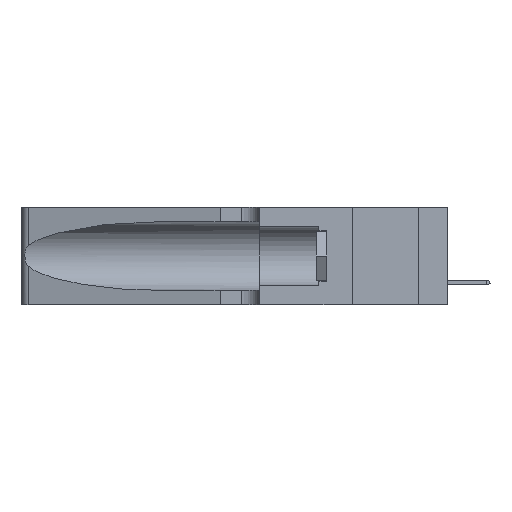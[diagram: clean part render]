
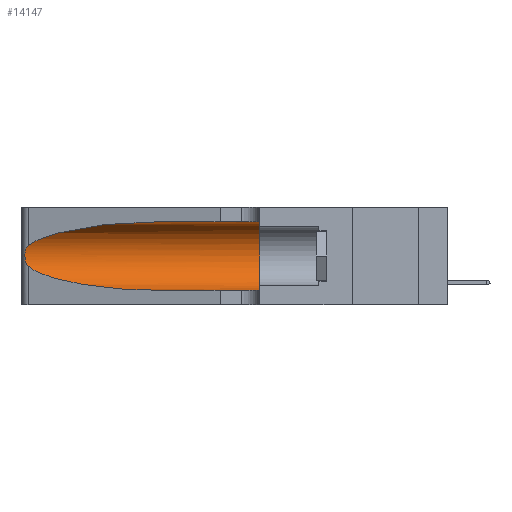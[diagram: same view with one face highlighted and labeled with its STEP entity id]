
A CAD part, left-side view. The second image highlights one B-rep face of the part: STEP entity #14147.
In plain terms, the highlighted cylindrical face has radius 3.308 mm (diameter 6.617 mm), a partial arc.
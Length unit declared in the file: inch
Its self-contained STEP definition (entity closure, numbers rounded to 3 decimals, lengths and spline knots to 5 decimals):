
#588 = VERTEX_POINT ( 'NONE', #4033 ) ;
#1008 = AXIS2_PLACEMENT_3D ( 'NONE', #1620, #20539, #9808 ) ;
#1588 = CARTESIAN_POINT ( 'NONE',  ( 0.18966, 0.96281, 0.05475 ) ) ;
#1620 = CARTESIAN_POINT ( 'NONE',  ( 0.1305, 1.61858, 0.185 ) ) ;
#1772 = ORIENTED_EDGE ( 'NONE', *, *, #20546, .T. ) ;
#1859 = EDGE_LOOP ( 'NONE', ( #26863, #9785, #7416, #1772, #9924, #25585 ) ) ;
#1901 = EDGE_CURVE ( 'NONE', #8899, #8452, #25184, .T. ) ;
#2953 = CARTESIAN_POINT ( 'NONE',  ( 0.25487, 1.22718, 0.22369 ) ) ;
#4033 = CARTESIAN_POINT ( 'NONE',  ( 0.1305, 0.35, 0.05475 ) ) ;
#4034 = VERTEX_POINT ( 'NONE', #15473 ) ;
#4769 = DIRECTION ( 'NONE',  ( 0., -1., 0. ) ) ;
#5078 = CARTESIAN_POINT ( 'NONE',  ( 0.25555, 1.22994, 0.2215 ) ) ;
#5127 = VECTOR ( 'NONE', #4769, 39.37008 ) ;
#5236 = DIRECTION ( 'NONE',  ( 0., 0., 1. ) ) ;
#5252 = CARTESIAN_POINT ( 'NONE',  ( 0.26075, 1.23896, 0.19203 ) ) ;
#5438 =( BOUNDED_CURVE ( )  B_SPLINE_CURVE ( 3, ( #11975, #26789, #1588, #12551 ),
 .UNSPECIFIED., .F., .T. ) 
 B_SPLINE_CURVE_WITH_KNOTS ( ( 4, 4 ),
 ( 3.44316, 4.71239 ),
 .UNSPECIFIED. ) 
 CURVE ( )  GEOMETRIC_REPRESENTATION_ITEM ( )  RATIONAL_B_SPLINE_CURVE ( ( 1., 0.87, 0.87, 1. ) ) 
 REPRESENTATION_ITEM ( '' )  );
#5460 = CARTESIAN_POINT ( 'NONE',  ( 0.25487, 1.22718, 0.22369 ) ) ;
#5530 = CARTESIAN_POINT ( 'NONE',  ( 0.25789, 1.23486, 0.15765 ) ) ;
#6013 = CARTESIAN_POINT ( 'NONE',  ( 0.25487, 1.22718, 0.22369 ) ) ;
#6825 = CARTESIAN_POINT ( 'NONE',  ( 0.1305, 0.72297, 0.05475 ) ) ;
#7416 = ORIENTED_EDGE ( 'NONE', *, *, #7505, .T. ) ;
#7505 = EDGE_CURVE ( 'NONE', #4034, #18145, #5438, .T. ) ;
#7836 =( BOUNDED_CURVE ( )  B_SPLINE_CURVE ( 3, ( #18072, #12247, #9733, #5460 ),
 .UNSPECIFIED., .F., .F. ) 
 B_SPLINE_CURVE_WITH_KNOTS ( ( 4, 4 ),
 ( 1.5708, 2.84003 ),
 .UNSPECIFIED. ) 
 CURVE ( )  GEOMETRIC_REPRESENTATION_ITEM ( )  RATIONAL_B_SPLINE_CURVE ( ( 1., 0.87, 0.87, 1. ) ) 
 REPRESENTATION_ITEM ( '' )  );
#8098 = CARTESIAN_POINT ( 'NONE',  ( 0.1305, 1.61858, 0.31525 ) ) ;
#8452 = VERTEX_POINT ( 'NONE', #18355 ) ;
#8899 = VERTEX_POINT ( 'NONE', #20578 ) ;
#9327 = CARTESIAN_POINT ( 'NONE',  ( 0.26018, 1.23835, 0.19895 ) ) ;
#9733 = CARTESIAN_POINT ( 'NONE',  ( 0.2373, 1.15595, 0.28018 ) ) ;
#9785 = ORIENTED_EDGE ( 'NONE', *, *, #19015, .T. ) ;
#9808 = DIRECTION ( 'NONE',  ( 0., 0., -1. ) ) ;
#9924 = ORIENTED_EDGE ( 'NONE', *, *, #17853, .F. ) ;
#11975 = CARTESIAN_POINT ( 'NONE',  ( 0.25487, 1.22718, 0.14631 ) ) ;
#12247 = CARTESIAN_POINT ( 'NONE',  ( 0.18966, 0.96281, 0.31525 ) ) ;
#12551 = CARTESIAN_POINT ( 'NONE',  ( 0.1305, 0.72297, 0.05475 ) ) ;
#13292 = CARTESIAN_POINT ( 'NONE',  ( 0.1305, 1.61858, 0.05475 ) ) ;
#13763 = CARTESIAN_POINT ( 'NONE',  ( 0.26017, 1.23833, 0.17102 ) ) ;
#14098 = DIRECTION ( 'NONE',  ( 0., -1., 0. ) ) ;
#14147 = ADVANCED_FACE ( 'NONE', ( #22108 ), #26999, .F. ) ;
#15473 = CARTESIAN_POINT ( 'NONE',  ( 0.25487, 1.22718, 0.14631 ) ) ;
#15841 = CARTESIAN_POINT ( 'NONE',  ( 0.25856, 1.23593, 0.16098 ) ) ;
#17234 = B_SPLINE_CURVE_WITH_KNOTS ( 'NONE', 3,
 ( #2953, #5078, #19810, #24023, #21923, #9327, #5252, #26278, #13763, #15841, #5530, #22568, #18411, #22476 ),
 .UNSPECIFIED., .F., .F.,
 ( 4, 2, 2, 2, 2, 2, 4 ),
 ( 0., 0.00027, 0.00053, 0.00107, 0.0016, 0.00187, 0.00214 ),
 .UNSPECIFIED. ) ;
#17290 = CIRCLE ( 'NONE', #20095, 0.13025 ) ;
#17853 = EDGE_CURVE ( 'NONE', #8452, #588, #17290, .T. ) ;
#18072 = CARTESIAN_POINT ( 'NONE',  ( 0.1305, 0.72297, 0.31525 ) ) ;
#18145 = VERTEX_POINT ( 'NONE', #6825 ) ;
#18355 = CARTESIAN_POINT ( 'NONE',  ( 0.1305, 0.35, 0.31525 ) ) ;
#18411 = CARTESIAN_POINT ( 'NONE',  ( 0.25555, 1.22993, 0.14849 ) ) ;
#19015 = EDGE_CURVE ( 'NONE', #24455, #4034, #17234, .T. ) ;
#19283 = LINE ( 'NONE', #13292, #5127 ) ;
#19498 = EDGE_CURVE ( 'NONE', #8899, #24455, #7836, .T. ) ;
#19606 = VECTOR ( 'NONE', #14098, 39.37008 ) ;
#19810 = CARTESIAN_POINT ( 'NONE',  ( 0.25639, 1.23184, 0.21858 ) ) ;
#20095 = AXIS2_PLACEMENT_3D ( 'NONE', #23919, #25983, #5236 ) ;
#20539 = DIRECTION ( 'NONE',  ( 0., -1., 0. ) ) ;
#20546 = EDGE_CURVE ( 'NONE', #18145, #588, #19283, .T. ) ;
#20578 = CARTESIAN_POINT ( 'NONE',  ( 0.1305, 0.72297, 0.31525 ) ) ;
#21923 = CARTESIAN_POINT ( 'NONE',  ( 0.25854, 1.2359, 0.20912 ) ) ;
#22108 = FACE_OUTER_BOUND ( 'NONE', #1859, .T. ) ;
#22476 = CARTESIAN_POINT ( 'NONE',  ( 0.25487, 1.22718, 0.14631 ) ) ;
#22568 = CARTESIAN_POINT ( 'NONE',  ( 0.25639, 1.23186, 0.15144 ) ) ;
#23919 = CARTESIAN_POINT ( 'NONE',  ( 0.1305, 0.35, 0.185 ) ) ;
#24023 = CARTESIAN_POINT ( 'NONE',  ( 0.25787, 1.23484, 0.2124 ) ) ;
#24455 = VERTEX_POINT ( 'NONE', #6013 ) ;
#25184 = LINE ( 'NONE', #8098, #19606 ) ;
#25585 = ORIENTED_EDGE ( 'NONE', *, *, #1901, .F. ) ;
#25983 = DIRECTION ( 'NONE',  ( 0., 1., 0. ) ) ;
#26278 = CARTESIAN_POINT ( 'NONE',  ( 0.26075, 1.23896, 0.178 ) ) ;
#26789 = CARTESIAN_POINT ( 'NONE',  ( 0.2373, 1.15595, 0.08982 ) ) ;
#26863 = ORIENTED_EDGE ( 'NONE', *, *, #19498, .T. ) ;
#26999 = CYLINDRICAL_SURFACE ( 'NONE', #1008, 0.13025 ) ;
